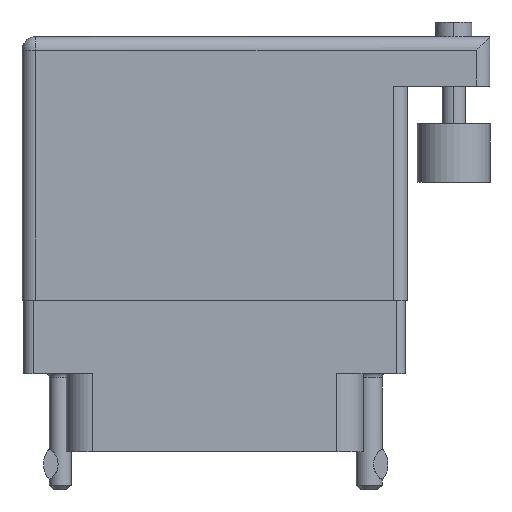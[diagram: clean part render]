
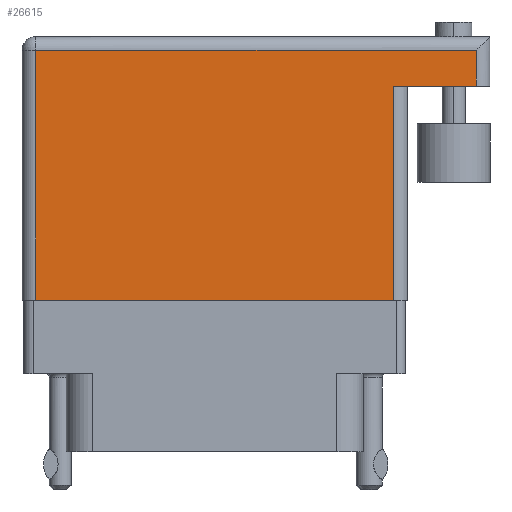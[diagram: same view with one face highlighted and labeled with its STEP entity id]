
A CAD part, front view. The second image highlights one B-rep face of the part: STEP entity #26615.
In plain terms, the highlighted face is planar.
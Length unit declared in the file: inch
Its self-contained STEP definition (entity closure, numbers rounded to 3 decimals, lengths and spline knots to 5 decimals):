
#530 = CARTESIAN_POINT ( 'NONE',  ( 0., 0.906, 0. ) ) ;
#612 = LINE ( 'NONE', #6284, #12405 ) ;
#1579 = VECTOR ( 'NONE', #17320, 39.37008 ) ;
#1989 = LINE ( 'NONE', #20043, #32268 ) ;
#3545 = ORIENTED_EDGE ( 'NONE', *, *, #14632, .T. ) ;
#3547 = DIRECTION ( 'NONE',  ( 1., 0., 0. ) ) ;
#4020 = VERTEX_POINT ( 'NONE', #17087 ) ;
#4810 = DIRECTION ( 'NONE',  ( 0., 1., 0. ) ) ;
#5585 = FACE_OUTER_BOUND ( 'NONE', #8030, .T. ) ;
#6284 = CARTESIAN_POINT ( 'NONE',  ( 0., 0.859, 0. ) ) ;
#6309 = CARTESIAN_POINT ( 'NONE',  ( 1.278, 0., 0. ) ) ;
#6489 = ORIENTED_EDGE ( 'NONE', *, *, #20309, .T. ) ;
#8030 = EDGE_LOOP ( 'NONE', ( #3545, #20714, #10074, #6489, #25978, #10193 ) ) ;
#8504 = DIRECTION ( 'NONE',  ( -1., 0., 0. ) ) ;
#10074 = ORIENTED_EDGE ( 'NONE', *, *, #17267, .F. ) ;
#10193 = ORIENTED_EDGE ( 'NONE', *, *, #16782, .T. ) ;
#12245 = CARTESIAN_POINT ( 'NONE',  ( 1.562, 0.906, 0. ) ) ;
#12405 = VECTOR ( 'NONE', #8504, 39.37008 ) ;
#13284 = PLANE ( 'NONE',  #14206 ) ;
#14206 = AXIS2_PLACEMENT_3D ( 'NONE', #530, #18143, #15816 ) ;
#14632 = EDGE_CURVE ( 'NONE', #18587, #18067, #28172, .T. ) ;
#15816 = DIRECTION ( 'NONE',  ( -1., 0., 0. ) ) ;
#16021 = VECTOR ( 'NONE', #3547, 39.37008 ) ;
#16665 = LINE ( 'NONE', #17633, #18254 ) ;
#16782 = EDGE_CURVE ( 'NONE', #18181, #18587, #22233, .T. ) ;
#17087 = CARTESIAN_POINT ( 'NONE',  ( 1.562, 0.736, 0. ) ) ;
#17267 = EDGE_CURVE ( 'NONE', #4020, #17949, #16665, .T. ) ;
#17320 = DIRECTION ( 'NONE',  ( 0., 1., 0. ) ) ;
#17633 = CARTESIAN_POINT ( 'NONE',  ( 1.609, 0.736, 0. ) ) ;
#17949 = VERTEX_POINT ( 'NONE', #18233 ) ;
#18067 = VERTEX_POINT ( 'NONE', #6309 ) ;
#18143 = DIRECTION ( 'NONE',  ( 0., 0., -1. ) ) ;
#18181 = VERTEX_POINT ( 'NONE', #21198 ) ;
#18233 = CARTESIAN_POINT ( 'NONE',  ( 1.278, 0.736, 0. ) ) ;
#18254 = VECTOR ( 'NONE', #25073, 39.37008 ) ;
#18587 = VERTEX_POINT ( 'NONE', #30577 ) ;
#18777 = CARTESIAN_POINT ( 'NONE',  ( 0., 0., 0. ) ) ;
#20043 = CARTESIAN_POINT ( 'NONE',  ( 1.278, 0.736, 0. ) ) ;
#20309 = EDGE_CURVE ( 'NONE', #4020, #30863, #20486, .T. ) ;
#20486 = LINE ( 'NONE', #12245, #1579 ) ;
#20714 = ORIENTED_EDGE ( 'NONE', *, *, #28027, .T. ) ;
#21198 = CARTESIAN_POINT ( 'NONE',  ( 0.047, 0.859, 0. ) ) ;
#22233 = LINE ( 'NONE', #25853, #30047 ) ;
#22656 = CARTESIAN_POINT ( 'NONE',  ( 1.562, 0.859, 0. ) ) ;
#23807 = EDGE_CURVE ( 'NONE', #30863, #18181, #612, .T. ) ;
#25073 = DIRECTION ( 'NONE',  ( -1., 0., 0. ) ) ;
#25853 = CARTESIAN_POINT ( 'NONE',  ( 0.047, 0., 0. ) ) ;
#25978 = ORIENTED_EDGE ( 'NONE', *, *, #23807, .T. ) ;
#26615 = ADVANCED_FACE ( 'NONE', ( #5585 ), #13284, .F. ) ;
#28027 = EDGE_CURVE ( 'NONE', #18067, #17949, #1989, .T. ) ;
#28172 = LINE ( 'NONE', #18777, #16021 ) ;
#30047 = VECTOR ( 'NONE', #30906, 39.37008 ) ;
#30577 = CARTESIAN_POINT ( 'NONE',  ( 0.047, 0., 0. ) ) ;
#30863 = VERTEX_POINT ( 'NONE', #22656 ) ;
#30906 = DIRECTION ( 'NONE',  ( 0., -1., 0. ) ) ;
#32268 = VECTOR ( 'NONE', #4810, 39.37008 ) ;
